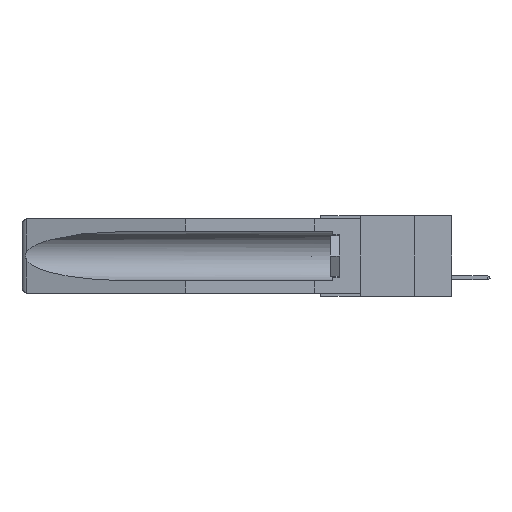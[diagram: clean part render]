
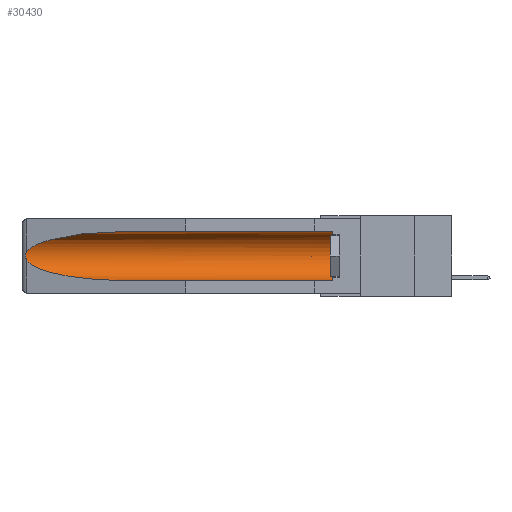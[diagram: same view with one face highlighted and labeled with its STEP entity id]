
A CAD part, left-side view. The second image highlights one B-rep face of the part: STEP entity #30430.
In plain terms, the highlighted cylindrical face has radius 2.857 mm (diameter 5.715 mm), a partial arc.
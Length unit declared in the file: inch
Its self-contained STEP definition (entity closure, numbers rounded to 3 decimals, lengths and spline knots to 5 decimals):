
#248 = EDGE_CURVE ( 'NONE', #15737, #30593, #23085, .T. ) ;
#431 = CIRCLE ( 'NONE', #31861, 0.1125 ) ;
#773 = EDGE_CURVE ( 'NONE', #30593, #13628, #26043, .T. ) ;
#1764 = CARTESIAN_POINT ( 'NONE',  ( 0.155, -0.30754, -0.1715 ) ) ;
#2300 = CARTESIAN_POINT ( 'NONE',  ( 0.26537, 1.52718, -0.14972 ) ) ;
#3430 = VECTOR ( 'NONE', #10237, 39.37008 ) ;
#3831 = CARTESIAN_POINT ( 'NONE',  ( 0.155, 0.126, -0.059 ) ) ;
#4410 = CARTESIAN_POINT ( 'NONE',  ( 0.155, 1.07973, -0.284 ) ) ;
#4976 = EDGE_CURVE ( 'NONE', #22605, #32430, #25563, .T. ) ;
#5095 = CARTESIAN_POINT ( 'NONE',  ( 0.155, -0.30754, -0.059 ) ) ;
#6864 = ORIENTED_EDGE ( 'NONE', *, *, #773, .T. ) ;
#7504 = VECTOR ( 'NONE', #30771, 39.37008 ) ;
#8678 = CARTESIAN_POINT ( 'NONE',  ( 0.21114, 1.30732, -0.059 ) ) ;
#9587 = LINE ( 'NONE', #28591, #7504 ) ;
#9591 = CARTESIAN_POINT ( 'NONE',  ( 0.155, 1.07973, -0.284 ) ) ;
#10237 = DIRECTION ( 'NONE',  ( 0., 1., 0. ) ) ;
#10502 = CYLINDRICAL_SURFACE ( 'NONE', #15843, 0.1125 ) ;
#10504 = DIRECTION ( 'NONE',  ( 0., -1., 0. ) ) ;
#12828 = CARTESIAN_POINT ( 'NONE',  ( 0.2673, 1.53269, -0.17917 ) ) ;
#13065 = CARTESIAN_POINT ( 'NONE',  ( 0.26597, 1.5296, -0.19026 ) ) ;
#13628 = VERTEX_POINT ( 'NONE', #23812 ) ;
#15473 = EDGE_CURVE ( 'NONE', #25428, #15737, #431, .T. ) ;
#15491 = CARTESIAN_POINT ( 'NONE',  ( 0.26537, 1.52718, -0.19328 ) ) ;
#15558 = CARTESIAN_POINT ( 'NONE',  ( 0.26537, 1.52718, -0.19328 ) ) ;
#15587 = ORIENTED_EDGE ( 'NONE', *, *, #4976, .T. ) ;
#15598 = CARTESIAN_POINT ( 'NONE',  ( 0.26655, 1.53094, -0.18657 ) ) ;
#15737 = VERTEX_POINT ( 'NONE', #3831 ) ;
#15833 = CARTESIAN_POINT ( 'NONE',  ( 0.2675, 1.53308, -0.17534 ) ) ;
#15843 = AXIS2_PLACEMENT_3D ( 'NONE', #1764, #22245, #25194 ) ;
#16365 = CARTESIAN_POINT ( 'NONE',  ( 0.26537, 1.52718, -0.14972 ) ) ;
#17336 = CARTESIAN_POINT ( 'NONE',  ( 0.21114, 1.30732, -0.284 ) ) ;
#17478 = FACE_OUTER_BOUND ( 'NONE', #18566, .T. ) ;
#17568 = CARTESIAN_POINT ( 'NONE',  ( 0.26537, 1.52718, -0.19328 ) ) ;
#18014 = B_SPLINE_CURVE_WITH_KNOTS ( 'NONE', 3,
 ( #2300, #20832, #28795, #33860, #31086, #15833, #12828, #15598, #13065, #15491 ),
 .UNSPECIFIED., .F., .F.,
 ( 4, 2, 2, 2, 4 ),
 ( 0., 0.00029, 0.00058, 0.00087, 0.00117 ),
 .UNSPECIFIED. ) ;
#18566 = EDGE_LOOP ( 'NONE', ( #6864, #33043, #15587, #29249, #23501, #23821 ) ) ;
#20630 = CARTESIAN_POINT ( 'NONE',  ( 0.155, 1.07973, -0.059 ) ) ;
#20832 = CARTESIAN_POINT ( 'NONE',  ( 0.26597, 1.52961, -0.15275 ) ) ;
#22245 = DIRECTION ( 'NONE',  ( 0., 1., 0. ) ) ;
#22605 = VERTEX_POINT ( 'NONE', #15558 ) ;
#23085 = LINE ( 'NONE', #5095, #3430 ) ;
#23501 = ORIENTED_EDGE ( 'NONE', *, *, #15473, .T. ) ;
#23812 = CARTESIAN_POINT ( 'NONE',  ( 0.26537, 1.52718, -0.14972 ) ) ;
#23821 = ORIENTED_EDGE ( 'NONE', *, *, #248, .T. ) ;
#25194 = DIRECTION ( 'NONE',  ( 0., 0., 1. ) ) ;
#25428 = VERTEX_POINT ( 'NONE', #33456 ) ;
#25563 =( BOUNDED_CURVE ( )  B_SPLINE_CURVE ( 3, ( #17568, #27924, #17336, #4410 ),
 .UNSPECIFIED., .F., .F. ) 
 B_SPLINE_CURVE_WITH_KNOTS ( ( 4, 4 ),
 ( 0.1948, 1.5708 ),
 .UNSPECIFIED. ) 
 CURVE ( )  GEOMETRIC_REPRESENTATION_ITEM ( )  RATIONAL_B_SPLINE_CURVE ( ( 1., 0.848, 0.848, 1. ) ) 
 REPRESENTATION_ITEM ( '' )  );
#25795 = DIRECTION ( 'NONE',  ( 0., 0., 1. ) ) ;
#26043 =( BOUNDED_CURVE ( )  B_SPLINE_CURVE ( 3, ( #29096, #8678, #31974, #16365 ),
 .UNSPECIFIED., .F., .F. ) 
 B_SPLINE_CURVE_WITH_KNOTS ( ( 4, 4 ),
 ( 4.71239, 6.08839 ),
 .UNSPECIFIED. ) 
 CURVE ( )  GEOMETRIC_REPRESENTATION_ITEM ( )  RATIONAL_B_SPLINE_CURVE ( ( 1., 0.848, 0.848, 1. ) ) 
 REPRESENTATION_ITEM ( '' )  );
#26119 = CARTESIAN_POINT ( 'NONE',  ( 0.155, 0.126, -0.1715 ) ) ;
#26128 = EDGE_CURVE ( 'NONE', #25428, #32430, #9587, .T. ) ;
#27742 = EDGE_CURVE ( 'NONE', #13628, #22605, #18014, .T. ) ;
#27924 = CARTESIAN_POINT ( 'NONE',  ( 0.25451, 1.48313, -0.24835 ) ) ;
#28591 = CARTESIAN_POINT ( 'NONE',  ( 0.155, -0.30754, -0.284 ) ) ;
#28795 = CARTESIAN_POINT ( 'NONE',  ( 0.26654, 1.53092, -0.15636 ) ) ;
#29096 = CARTESIAN_POINT ( 'NONE',  ( 0.155, 1.07973, -0.059 ) ) ;
#29249 = ORIENTED_EDGE ( 'NONE', *, *, #26128, .F. ) ;
#30430 = ADVANCED_FACE ( 'NONE', ( #17478 ), #10502, .F. ) ;
#30593 = VERTEX_POINT ( 'NONE', #20630 ) ;
#30771 = DIRECTION ( 'NONE',  ( 0., 1., 0. ) ) ;
#31086 = CARTESIAN_POINT ( 'NONE',  ( 0.2675, 1.53308, -0.16763 ) ) ;
#31861 = AXIS2_PLACEMENT_3D ( 'NONE', #26119, #10504, #25795 ) ;
#31974 = CARTESIAN_POINT ( 'NONE',  ( 0.25451, 1.48313, -0.09465 ) ) ;
#32430 = VERTEX_POINT ( 'NONE', #9591 ) ;
#33043 = ORIENTED_EDGE ( 'NONE', *, *, #27742, .T. ) ;
#33456 = CARTESIAN_POINT ( 'NONE',  ( 0.155, 0.126, -0.284 ) ) ;
#33860 = CARTESIAN_POINT ( 'NONE',  ( 0.2673, 1.5327, -0.16383 ) ) ;
